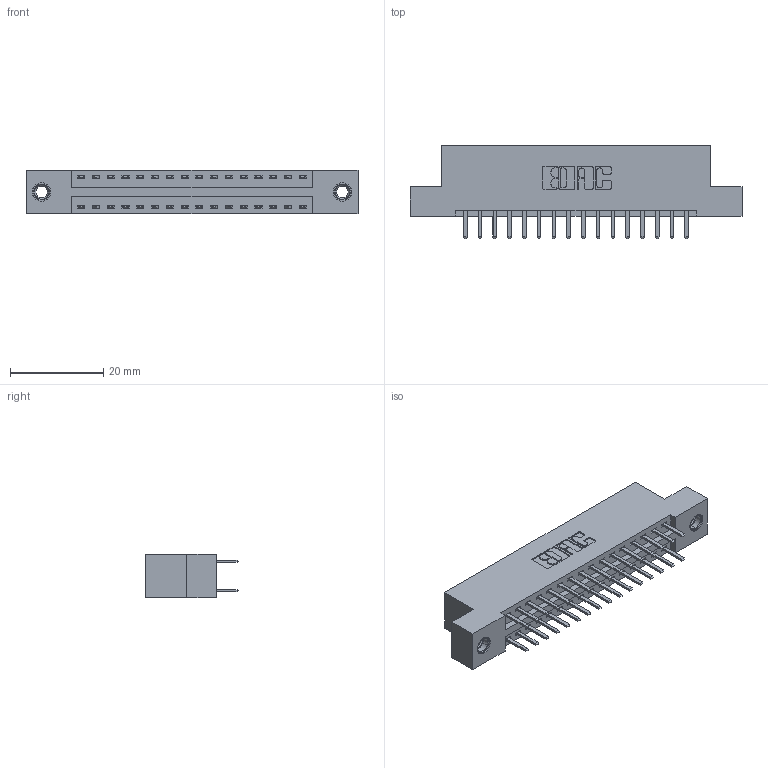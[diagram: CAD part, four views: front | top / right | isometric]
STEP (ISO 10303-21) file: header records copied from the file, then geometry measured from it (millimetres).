
FILE_DESCRIPTION (( 'STEP AP203' ), '1' );
FILE_NAME ('396-032-520-207.STEP', '2018-09-05T09:43:09', ( '' ), ( '' ), 'SwSTEP 2.0', 'SolidWorks 2016', '' );
FILE_SCHEMA (( 'CONFIG_CONTROL_DESIGN' ));
Length unit declared in the file: inch
Products named in the file (4): 396-032-520-207; 346 Part_Flush Mounting Lugs - 0.156 Dia-TI; 345-292-001_345-293-120; 345-250-001_345-250-005-103
Assembly tree (35 placements, depth 2):
  396-032-520-207
    346 Part_Flush Mounting Lugs - 0.156 Dia-TI
    345-292-001_345-293-120  x32
    345-250-001_345-250-005-103  x2
Bounding box: 71.37 x 20.02 x 9.4 mm (x, y, z)
Volume: 6730.3 mm3; surface area: 8843.4 mm2
Topology: 35 solids, 35 shells, 1974 faces, 5681 edges, 3694 vertices
Faces by surface type: plane 1292, cylinder 666, cone 12, torus 4
Entity records: 15242 total; most frequent: CARTESIAN_POINT 2543, ORIENTED_EDGE 2458, DIRECTION 2307, EDGE_CURVE 1229, LINE 1009, VECTOR 1009, VERTEX_POINT 812, AXIS2_PLACEMENT_3D 649
